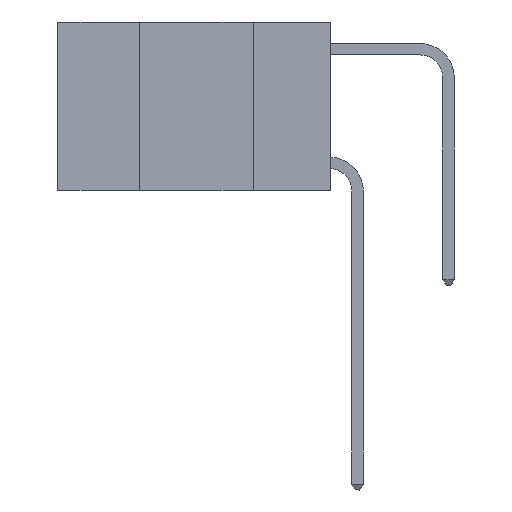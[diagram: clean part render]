
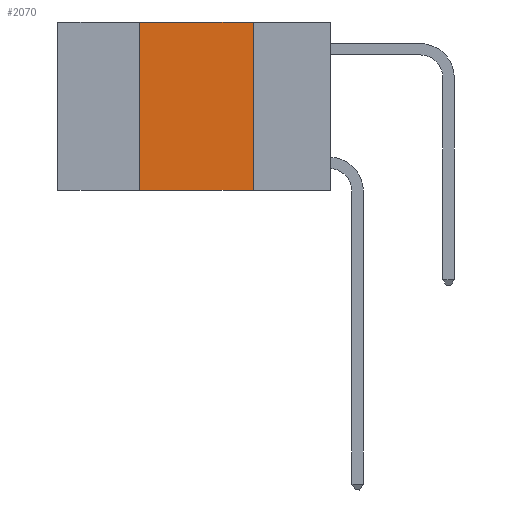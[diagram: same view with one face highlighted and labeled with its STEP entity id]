
A CAD part, left-side view. The second image highlights one B-rep face of the part: STEP entity #2070.
In plain terms, the highlighted planar face has unit normal (-1, 0, 0).
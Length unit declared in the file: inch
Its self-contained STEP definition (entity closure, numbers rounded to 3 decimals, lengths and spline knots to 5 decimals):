
#293 = EDGE_CURVE ( 'NONE', #1003, #3744, #23710, .T. ) ;
#531 = CARTESIAN_POINT ( 'NONE',  ( 0., 0.17, -0.37 ) ) ;
#1003 = VERTEX_POINT ( 'NONE', #21513 ) ;
#1470 = AXIS2_PLACEMENT_3D ( 'NONE', #3041, #10702, #12855 ) ;
#2070 = ADVANCED_FACE ( 'NONE', ( #3802 ), #8914, .F. ) ;
#2837 = LINE ( 'NONE', #11695, #24175 ) ;
#3041 = CARTESIAN_POINT ( 'NONE',  ( 0., 0.6, 0. ) ) ;
#3744 = VERTEX_POINT ( 'NONE', #16100 ) ;
#3802 = FACE_OUTER_BOUND ( 'NONE', #15016, .T. ) ;
#4541 = VERTEX_POINT ( 'NONE', #531 ) ;
#4880 = DIRECTION ( 'NONE',  ( 0., -1., 0. ) ) ;
#6306 = LINE ( 'NONE', #10094, #8150 ) ;
#7366 = ORIENTED_EDGE ( 'NONE', *, *, #14525, .F. ) ;
#8150 = VECTOR ( 'NONE', #23702, 39.37008 ) ;
#8914 = PLANE ( 'NONE',  #1470 ) ;
#9089 = VECTOR ( 'NONE', #4880, 39.37008 ) ;
#9446 = CARTESIAN_POINT ( 'NONE',  ( 0., 0.42, 0. ) ) ;
#10094 = CARTESIAN_POINT ( 'NONE',  ( 0., 0.17, 0. ) ) ;
#10702 = DIRECTION ( 'NONE',  ( 1., 0., 0. ) ) ;
#10819 = ORIENTED_EDGE ( 'NONE', *, *, #11734, .T. ) ;
#11395 = DIRECTION ( 'NONE',  ( 0., 0., 1. ) ) ;
#11695 = CARTESIAN_POINT ( 'NONE',  ( 0., 0.6, -0.37 ) ) ;
#11734 = EDGE_CURVE ( 'NONE', #1003, #4541, #2837, .T. ) ;
#12855 = DIRECTION ( 'NONE',  ( 0., 0., -1. ) ) ;
#13669 = ORIENTED_EDGE ( 'NONE', *, *, #20209, .F. ) ;
#13983 = CARTESIAN_POINT ( 'NONE',  ( 0., 0.17, 0. ) ) ;
#14525 = EDGE_CURVE ( 'NONE', #3744, #20889, #17325, .T. ) ;
#15016 = EDGE_LOOP ( 'NONE', ( #13669, #7366, #16712, #10819 ) ) ;
#15842 = DIRECTION ( 'NONE',  ( 0., -1., 0. ) ) ;
#16100 = CARTESIAN_POINT ( 'NONE',  ( 0., 0.42, 0. ) ) ;
#16712 = ORIENTED_EDGE ( 'NONE', *, *, #293, .F. ) ;
#17325 = LINE ( 'NONE', #20281, #9089 ) ;
#20209 = EDGE_CURVE ( 'NONE', #20889, #4541, #6306, .T. ) ;
#20281 = CARTESIAN_POINT ( 'NONE',  ( 0., 0.6, 0. ) ) ;
#20889 = VERTEX_POINT ( 'NONE', #13983 ) ;
#20994 = VECTOR ( 'NONE', #11395, 39.37008 ) ;
#21513 = CARTESIAN_POINT ( 'NONE',  ( 0., 0.42, -0.37 ) ) ;
#23702 = DIRECTION ( 'NONE',  ( 0., 0., -1. ) ) ;
#23710 = LINE ( 'NONE', #9446, #20994 ) ;
#24175 = VECTOR ( 'NONE', #15842, 39.37008 ) ;
